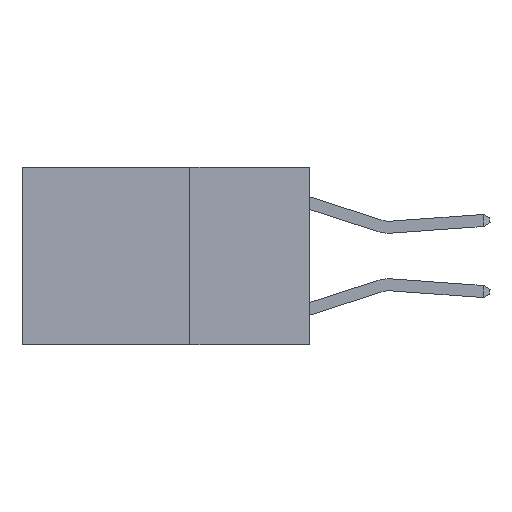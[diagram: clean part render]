
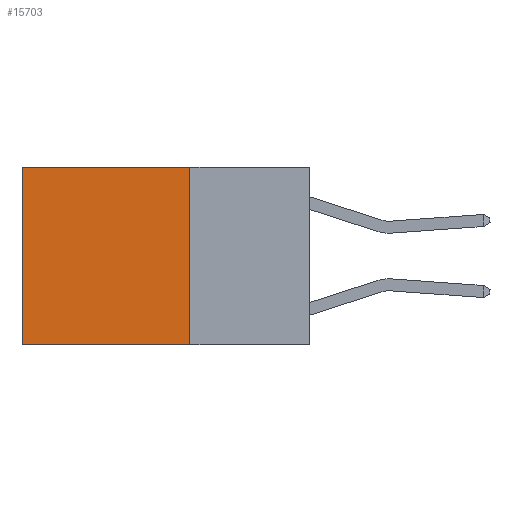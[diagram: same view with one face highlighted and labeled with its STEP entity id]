
A CAD part, left-side view. The second image highlights one B-rep face of the part: STEP entity #15703.
In plain terms, the highlighted planar face has unit normal (-1, 0, 0).
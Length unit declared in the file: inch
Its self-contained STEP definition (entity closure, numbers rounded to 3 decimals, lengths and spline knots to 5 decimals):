
#457 = CARTESIAN_POINT ( 'NONE',  ( 0.2625, 0.25, 0. ) ) ;
#1388 = LINE ( 'NONE', #26201, #23577 ) ;
#2288 = EDGE_CURVE ( 'NONE', #11516, #13098, #1388, .T. ) ;
#3343 = CARTESIAN_POINT ( 'NONE',  ( 0.2625, 0.6, 0. ) ) ;
#3551 = CARTESIAN_POINT ( 'NONE',  ( 0.2625, 0.6, -0.37 ) ) ;
#3887 = VECTOR ( 'NONE', #20626, 39.37008 ) ;
#5315 = DIRECTION ( 'NONE',  ( 0., 1., 0. ) ) ;
#5579 = EDGE_LOOP ( 'NONE', ( #7869, #10331, #24109, #28794 ) ) ;
#5808 = CARTESIAN_POINT ( 'NONE',  ( 0.2625, 0.25, 0. ) ) ;
#7049 = LINE ( 'NONE', #15993, #17714 ) ;
#7210 = VERTEX_POINT ( 'NONE', #17041 ) ;
#7869 = ORIENTED_EDGE ( 'NONE', *, *, #22003, .T. ) ;
#8433 = PLANE ( 'NONE',  #21045 ) ;
#9719 = EDGE_CURVE ( 'NONE', #11516, #7210, #27306, .T. ) ;
#10331 = ORIENTED_EDGE ( 'NONE', *, *, #19119, .F. ) ;
#11516 = VERTEX_POINT ( 'NONE', #19382 ) ;
#13098 = VERTEX_POINT ( 'NONE', #13478 ) ;
#13478 = CARTESIAN_POINT ( 'NONE',  ( 0.2625, 0.25, -0.37 ) ) ;
#14167 = LINE ( 'NONE', #3343, #3887 ) ;
#14744 = DIRECTION ( 'NONE',  ( 1., 0., 0. ) ) ;
#15703 = ADVANCED_FACE ( 'NONE', ( #28549 ), #8433, .F. ) ;
#15993 = CARTESIAN_POINT ( 'NONE',  ( 0.2625, 0.25, -0.37 ) ) ;
#16134 = DIRECTION ( 'NONE',  ( 0., 1., 0. ) ) ;
#17041 = CARTESIAN_POINT ( 'NONE',  ( 0.2625, 0.6, 0. ) ) ;
#17364 = VERTEX_POINT ( 'NONE', #3551 ) ;
#17714 = VECTOR ( 'NONE', #16134, 39.37008 ) ;
#19119 = EDGE_CURVE ( 'NONE', #13098, #17364, #7049, .T. ) ;
#19382 = CARTESIAN_POINT ( 'NONE',  ( 0.2625, 0.25, 0. ) ) ;
#19724 = VECTOR ( 'NONE', #5315, 39.37008 ) ;
#20626 = DIRECTION ( 'NONE',  ( 0., 0., -1. ) ) ;
#21045 = AXIS2_PLACEMENT_3D ( 'NONE', #5808, #14744, #23698 ) ;
#21770 = DIRECTION ( 'NONE',  ( 0., 0., -1. ) ) ;
#22003 = EDGE_CURVE ( 'NONE', #7210, #17364, #14167, .T. ) ;
#23577 = VECTOR ( 'NONE', #21770, 39.37008 ) ;
#23698 = DIRECTION ( 'NONE',  ( 0., 0., -1. ) ) ;
#24109 = ORIENTED_EDGE ( 'NONE', *, *, #2288, .F. ) ;
#26201 = CARTESIAN_POINT ( 'NONE',  ( 0.2625, 0.25, 0. ) ) ;
#27306 = LINE ( 'NONE', #457, #19724 ) ;
#28549 = FACE_OUTER_BOUND ( 'NONE', #5579, .T. ) ;
#28794 = ORIENTED_EDGE ( 'NONE', *, *, #9719, .T. ) ;
